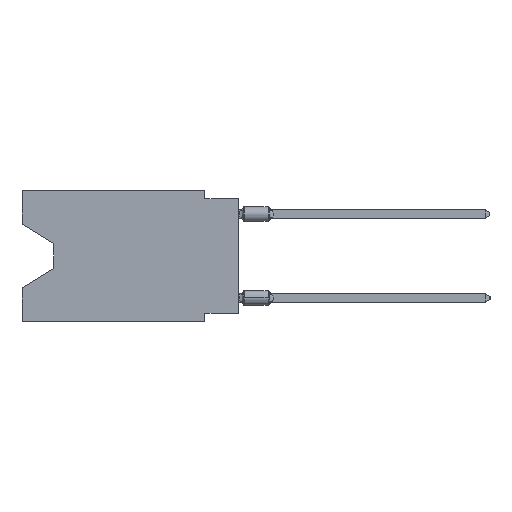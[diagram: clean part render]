
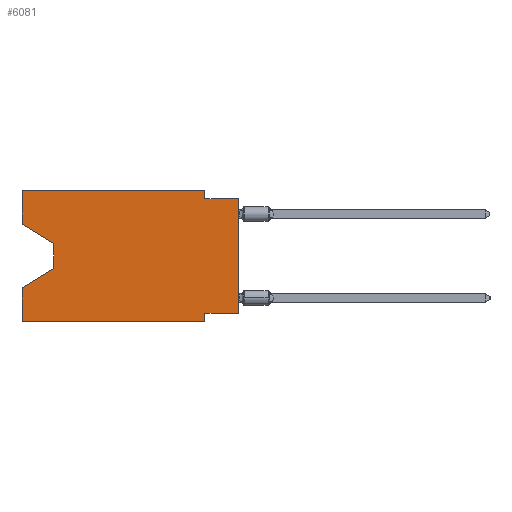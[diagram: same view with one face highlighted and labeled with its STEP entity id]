
A CAD part, left-side view. The second image highlights one B-rep face of the part: STEP entity #6081.
In plain terms, the highlighted planar face has unit normal (-1, 0, 0).
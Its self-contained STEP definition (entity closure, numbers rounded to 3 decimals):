
#247 = CARTESIAN_POINT ( 'NONE',  ( 0., 0., 0. ) ) ;
#518 = VERTEX_POINT ( 'NONE', #13610 ) ;
#751 = VECTOR ( 'NONE', #15893, 1000. ) ;
#1316 = EDGE_CURVE ( 'NONE', #8575, #15044, #8833, .T. ) ;
#2654 = VERTEX_POINT ( 'NONE', #29506 ) ;
#3300 = CARTESIAN_POINT ( 'NONE',  ( 0., 16.383, 0. ) ) ;
#4947 = VECTOR ( 'NONE', #26248, 1000. ) ;
#5107 = CARTESIAN_POINT ( 'NONE',  ( 0., 13.97, -5.893 ) ) ;
#5181 = CARTESIAN_POINT ( 'NONE',  ( 0., 13.97, -4.013 ) ) ;
#5376 = VECTOR ( 'NONE', #11701, 1000. ) ;
#6081 = ADVANCED_FACE ( 'NONE', ( #25897 ), #30922, .F. ) ;
#6168 = DIRECTION ( 'NONE',  ( 0., -1., 0. ) ) ;
#6169 = LINE ( 'NONE', #247, #20255 ) ;
#6333 = CARTESIAN_POINT ( 'NONE',  ( 0., 0., -0.635 ) ) ;
#6395 = VERTEX_POINT ( 'NONE', #6333 ) ;
#6745 = VECTOR ( 'NONE', #19996, 1000. ) ;
#6974 = ORIENTED_EDGE ( 'NONE', *, *, #17808, .T. ) ;
#7624 = ORIENTED_EDGE ( 'NONE', *, *, #23010, .F. ) ;
#7664 = VERTEX_POINT ( 'NONE', #14364 ) ;
#7757 = LINE ( 'NONE', #20838, #23852 ) ;
#8467 = DIRECTION ( 'NONE',  ( 0., 0., -1. ) ) ;
#8575 = VERTEX_POINT ( 'NONE', #9825 ) ;
#8833 = LINE ( 'NONE', #17248, #26455 ) ;
#8839 = CARTESIAN_POINT ( 'NONE',  ( 0., 16.383, -9.906 ) ) ;
#9038 = LINE ( 'NONE', #8839, #5376 ) ;
#9825 = CARTESIAN_POINT ( 'NONE',  ( 0., 16.383, -2.546 ) ) ;
#10763 = ORIENTED_EDGE ( 'NONE', *, *, #26298, .F. ) ;
#10934 = CARTESIAN_POINT ( 'NONE',  ( 0., 0., -0.635 ) ) ;
#11199 = VECTOR ( 'NONE', #6168, 1000. ) ;
#11366 = DIRECTION ( 'NONE',  ( 0., 0., 1. ) ) ;
#11635 = VERTEX_POINT ( 'NONE', #23767 ) ;
#11701 = DIRECTION ( 'NONE',  ( 0., -1., 0. ) ) ;
#11723 = ORIENTED_EDGE ( 'NONE', *, *, #21725, .F. ) ;
#11773 = ORIENTED_EDGE ( 'NONE', *, *, #21786, .F. ) ;
#12819 = ORIENTED_EDGE ( 'NONE', *, *, #1316, .T. ) ;
#12924 = VERTEX_POINT ( 'NONE', #18215 ) ;
#13610 = CARTESIAN_POINT ( 'NONE',  ( 0., 13.97, -5.893 ) ) ;
#14182 = VERTEX_POINT ( 'NONE', #34898 ) ;
#14364 = CARTESIAN_POINT ( 'NONE',  ( 0., 0., -9.271 ) ) ;
#14574 = AXIS2_PLACEMENT_3D ( 'NONE', #33609, #28412, #22888 ) ;
#14979 = CARTESIAN_POINT ( 'NONE',  ( 0., 2.54, -0.635 ) ) ;
#15044 = VERTEX_POINT ( 'NONE', #5181 ) ;
#15794 = ORIENTED_EDGE ( 'NONE', *, *, #29679, .F. ) ;
#15893 = DIRECTION ( 'NONE',  ( 0., 0., -1. ) ) ;
#16772 = CARTESIAN_POINT ( 'NONE',  ( 0., 0., -9.271 ) ) ;
#17248 = CARTESIAN_POINT ( 'NONE',  ( 0., 16.383, -2.546 ) ) ;
#17368 = ORIENTED_EDGE ( 'NONE', *, *, #33760, .F. ) ;
#17808 = EDGE_CURVE ( 'NONE', #11635, #17907, #9038, .T. ) ;
#17846 = EDGE_CURVE ( 'NONE', #7664, #6395, #6169, .T. ) ;
#17907 = VERTEX_POINT ( 'NONE', #22123 ) ;
#18215 = CARTESIAN_POINT ( 'NONE',  ( 0., 16.383, -7.36 ) ) ;
#18260 = ORIENTED_EDGE ( 'NONE', *, *, #18410, .T. ) ;
#18410 = EDGE_CURVE ( 'NONE', #518, #12924, #18740, .T. ) ;
#18740 = LINE ( 'NONE', #5107, #33982 ) ;
#19782 = LINE ( 'NONE', #30696, #11199 ) ;
#19996 = DIRECTION ( 'NONE',  ( 0., 0., -1. ) ) ;
#20168 = DIRECTION ( 'NONE',  ( 0., 1., 0. ) ) ;
#20255 = VECTOR ( 'NONE', #11366, 1000. ) ;
#20452 = EDGE_CURVE ( 'NONE', #15044, #518, #7757, .T. ) ;
#20691 = CARTESIAN_POINT ( 'NONE',  ( 0., 2.54, -9.906 ) ) ;
#20838 = CARTESIAN_POINT ( 'NONE',  ( 0., 13.97, -4.013 ) ) ;
#20850 = VECTOR ( 'NONE', #20168, 1000. ) ;
#21530 = LINE ( 'NONE', #10934, #29513 ) ;
#21642 = VERTEX_POINT ( 'NONE', #14979 ) ;
#21725 = EDGE_CURVE ( 'NONE', #30443, #21642, #24285, .T. ) ;
#21786 = EDGE_CURVE ( 'NONE', #8575, #2654, #30881, .T. ) ;
#21862 = DIRECTION ( 'NONE',  ( 0., -1., 0. ) ) ;
#22123 = CARTESIAN_POINT ( 'NONE',  ( 0., 2.54, -9.906 ) ) ;
#22888 = DIRECTION ( 'NONE',  ( 0., 0., -1. ) ) ;
#22937 = CARTESIAN_POINT ( 'NONE',  ( 0., 2.54, 0. ) ) ;
#23010 = EDGE_CURVE ( 'NONE', #7664, #14182, #30915, .T. ) ;
#23767 = CARTESIAN_POINT ( 'NONE',  ( 0., 16.383, -9.906 ) ) ;
#23852 = VECTOR ( 'NONE', #8467, 1000. ) ;
#24285 = LINE ( 'NONE', #32334, #751 ) ;
#24738 = ORIENTED_EDGE ( 'NONE', *, *, #20452, .T. ) ;
#25897 = FACE_OUTER_BOUND ( 'NONE', #29796, .T. ) ;
#26248 = DIRECTION ( 'NONE',  ( 0., 0., 1. ) ) ;
#26298 = EDGE_CURVE ( 'NONE', #21642, #6395, #21530, .T. ) ;
#26455 = VECTOR ( 'NONE', #28153, 1000. ) ;
#28147 = ORIENTED_EDGE ( 'NONE', *, *, #17846, .T. ) ;
#28153 = DIRECTION ( 'NONE',  ( 0., -0.855, -0.519 ) ) ;
#28412 = DIRECTION ( 'NONE',  ( 1., 0., 0. ) ) ;
#28907 = LINE ( 'NONE', #20691, #6745 ) ;
#28909 = CARTESIAN_POINT ( 'NONE',  ( 0., 16.383, 0. ) ) ;
#29104 = LINE ( 'NONE', #28909, #4947 ) ;
#29506 = CARTESIAN_POINT ( 'NONE',  ( 0., 16.383, 0. ) ) ;
#29513 = VECTOR ( 'NONE', #21862, 1000. ) ;
#29603 = ORIENTED_EDGE ( 'NONE', *, *, #30263, .F. ) ;
#29679 = EDGE_CURVE ( 'NONE', #2654, #30443, #19782, .T. ) ;
#29796 = EDGE_LOOP ( 'NONE', ( #12819, #24738, #18260, #29603, #6974, #17368, #7624, #28147, #10763, #11723, #15794, #11773 ) ) ;
#30263 = EDGE_CURVE ( 'NONE', #11635, #12924, #29104, .T. ) ;
#30443 = VERTEX_POINT ( 'NONE', #22937 ) ;
#30696 = CARTESIAN_POINT ( 'NONE',  ( 0., 16.383, 0. ) ) ;
#30881 = LINE ( 'NONE', #3300, #33925 ) ;
#30915 = LINE ( 'NONE', #16772, #20850 ) ;
#30922 = PLANE ( 'NONE',  #14574 ) ;
#32334 = CARTESIAN_POINT ( 'NONE',  ( 0., 2.54, 0. ) ) ;
#32651 = DIRECTION ( 'NONE',  ( 0., 0.855, -0.519 ) ) ;
#33609 = CARTESIAN_POINT ( 'NONE',  ( 0., 16.383, 0. ) ) ;
#33726 = DIRECTION ( 'NONE',  ( 0., 0., 1. ) ) ;
#33760 = EDGE_CURVE ( 'NONE', #14182, #17907, #28907, .T. ) ;
#33925 = VECTOR ( 'NONE', #33726, 1000. ) ;
#33982 = VECTOR ( 'NONE', #32651, 1000. ) ;
#34898 = CARTESIAN_POINT ( 'NONE',  ( 0., 2.54, -9.271 ) ) ;
